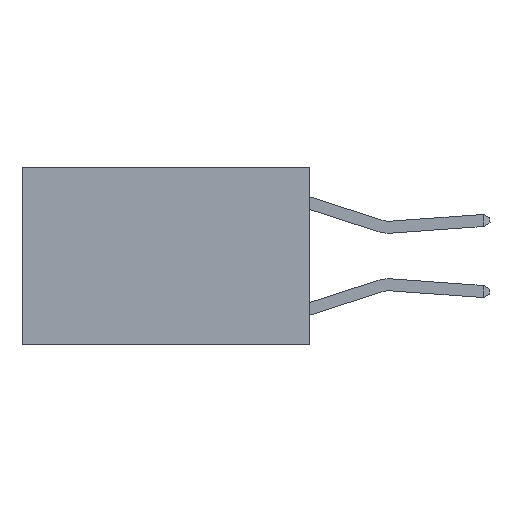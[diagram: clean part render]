
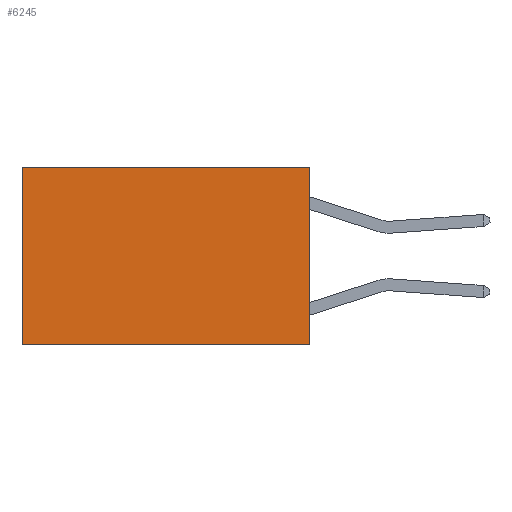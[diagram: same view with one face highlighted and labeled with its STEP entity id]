
A CAD part, left-side view. The second image highlights one B-rep face of the part: STEP entity #6245.
In plain terms, the highlighted planar face has unit normal (-1, 0, 0).
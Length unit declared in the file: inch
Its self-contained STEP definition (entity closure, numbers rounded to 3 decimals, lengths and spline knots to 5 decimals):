
#44 = VERTEX_POINT ( 'NONE', #7384 ) ;
#442 = DIRECTION ( 'NONE',  ( 0., 0., -1. ) ) ;
#805 = VERTEX_POINT ( 'NONE', #5432 ) ;
#2186 = LINE ( 'NONE', #5649, #4033 ) ;
#2215 = CARTESIAN_POINT ( 'NONE',  ( 0.2625, 0., -0.37 ) ) ;
#2402 = VECTOR ( 'NONE', #2873, 39.37008 ) ;
#2427 = DIRECTION ( 'NONE',  ( 0., 0., -1. ) ) ;
#2515 = LINE ( 'NONE', #2880, #7647 ) ;
#2873 = DIRECTION ( 'NONE',  ( 0., 1., 0. ) ) ;
#2880 = CARTESIAN_POINT ( 'NONE',  ( 0.2625, 0., 0. ) ) ;
#3459 = AXIS2_PLACEMENT_3D ( 'NONE', #5659, #6278, #2427 ) ;
#3470 = VERTEX_POINT ( 'NONE', #6519 ) ;
#3789 = ORIENTED_EDGE ( 'NONE', *, *, #5397, .T. ) ;
#4033 = VECTOR ( 'NONE', #4388, 39.37008 ) ;
#4039 = CARTESIAN_POINT ( 'NONE',  ( 0.2625, 0., 0. ) ) ;
#4388 = DIRECTION ( 'NONE',  ( 0., 0., -1. ) ) ;
#4469 = FACE_OUTER_BOUND ( 'NONE', #6020, .T. ) ;
#4717 = EDGE_CURVE ( 'NONE', #44, #805, #2186, .T. ) ;
#4780 = EDGE_CURVE ( 'NONE', #5146, #3470, #6937, .T. ) ;
#5022 = PLANE ( 'NONE',  #3459 ) ;
#5146 = VERTEX_POINT ( 'NONE', #4039 ) ;
#5397 = EDGE_CURVE ( 'NONE', #5146, #44, #2515, .T. ) ;
#5432 = CARTESIAN_POINT ( 'NONE',  ( 0.2625, 0.6, -0.37 ) ) ;
#5649 = CARTESIAN_POINT ( 'NONE',  ( 0.2625, 0.6, 0. ) ) ;
#5659 = CARTESIAN_POINT ( 'NONE',  ( 0.2625, 0., 0. ) ) ;
#5924 = ORIENTED_EDGE ( 'NONE', *, *, #6014, .F. ) ;
#6014 = EDGE_CURVE ( 'NONE', #3470, #805, #6035, .T. ) ;
#6020 = EDGE_LOOP ( 'NONE', ( #7961, #5924, #7674, #3789 ) ) ;
#6035 = LINE ( 'NONE', #2215, #2402 ) ;
#6097 = DIRECTION ( 'NONE',  ( 0., 1., 0. ) ) ;
#6245 = ADVANCED_FACE ( 'NONE', ( #4469 ), #5022, .F. ) ;
#6278 = DIRECTION ( 'NONE',  ( 1., 0., 0. ) ) ;
#6519 = CARTESIAN_POINT ( 'NONE',  ( 0.2625, 0., -0.37 ) ) ;
#6937 = LINE ( 'NONE', #8208, #8378 ) ;
#7384 = CARTESIAN_POINT ( 'NONE',  ( 0.2625, 0.6, 0. ) ) ;
#7647 = VECTOR ( 'NONE', #6097, 39.37008 ) ;
#7674 = ORIENTED_EDGE ( 'NONE', *, *, #4780, .F. ) ;
#7961 = ORIENTED_EDGE ( 'NONE', *, *, #4717, .T. ) ;
#8208 = CARTESIAN_POINT ( 'NONE',  ( 0.2625, 0., 0. ) ) ;
#8378 = VECTOR ( 'NONE', #442, 39.37008 ) ;
